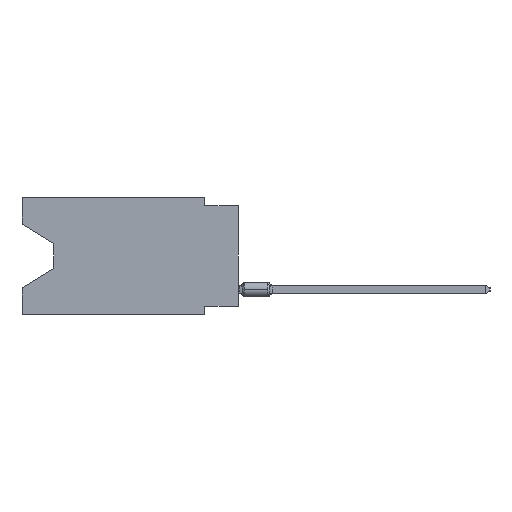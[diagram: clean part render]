
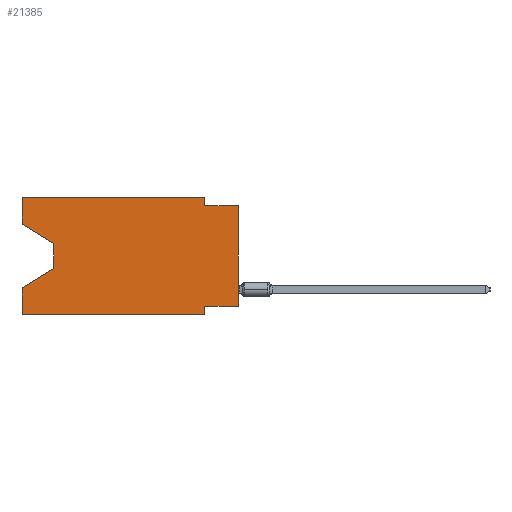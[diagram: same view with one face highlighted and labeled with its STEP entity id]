
A CAD part, left-side view. The second image highlights one B-rep face of the part: STEP entity #21385.
In plain terms, the highlighted planar face has unit normal (-1, 0, 0).
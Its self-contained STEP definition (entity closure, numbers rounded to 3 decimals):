
#199 = VECTOR ( 'NONE', #45842, 1000. ) ;
#416 = DIRECTION ( 'NONE',  ( 1., 0., 0. ) ) ;
#515 = ORIENTED_EDGE ( 'NONE', *, *, #51809, .F. ) ;
#555 = ORIENTED_EDGE ( 'NONE', *, *, #45054, .F. ) ;
#804 = CARTESIAN_POINT ( 'NONE',  ( 0., 16.383, 0. ) ) ;
#1162 = VERTEX_POINT ( 'NONE', #34680 ) ;
#1361 = DIRECTION ( 'NONE',  ( 0., 0., 1. ) ) ;
#1737 = EDGE_CURVE ( 'NONE', #40286, #1162, #40744, .T. ) ;
#2355 = VECTOR ( 'NONE', #50678, 1000. ) ;
#4151 = DIRECTION ( 'NONE',  ( 0., 0., -1. ) ) ;
#4203 = DIRECTION ( 'NONE',  ( 0., 0., 1. ) ) ;
#4494 = CARTESIAN_POINT ( 'NONE',  ( 0., 13.97, -5.385 ) ) ;
#4905 = CARTESIAN_POINT ( 'NONE',  ( 0., 2.54, -8.89 ) ) ;
#4946 = VECTOR ( 'NONE', #25974, 1000. ) ;
#4986 = CARTESIAN_POINT ( 'NONE',  ( 0., 2.54, -0.635 ) ) ;
#5326 = DIRECTION ( 'NONE',  ( 0., -1., 0. ) ) ;
#6406 = LINE ( 'NONE', #15173, #2355 ) ;
#9459 = VERTEX_POINT ( 'NONE', #20965 ) ;
#13341 = DIRECTION ( 'NONE',  ( 0., 1., 0. ) ) ;
#13420 = VERTEX_POINT ( 'NONE', #39479 ) ;
#13816 = LINE ( 'NONE', #26316, #24808 ) ;
#13938 = VECTOR ( 'NONE', #5326, 1000. ) ;
#14042 = EDGE_CURVE ( 'NONE', #21015, #50200, #6406, .T. ) ;
#14538 = CARTESIAN_POINT ( 'NONE',  ( 0., 13.97, -3.505 ) ) ;
#14725 = CARTESIAN_POINT ( 'NONE',  ( 0., 16.383, -8.89 ) ) ;
#15173 = CARTESIAN_POINT ( 'NONE',  ( 0., 13.97, -5.385 ) ) ;
#15688 = VERTEX_POINT ( 'NONE', #4986 ) ;
#15832 = VERTEX_POINT ( 'NONE', #14538 ) ;
#15868 = CARTESIAN_POINT ( 'NONE',  ( 0., 16.383, 0. ) ) ;
#16449 = CARTESIAN_POINT ( 'NONE',  ( 0., 0., 0. ) ) ;
#17050 = DIRECTION ( 'NONE',  ( 0., -1., 0. ) ) ;
#17174 = VECTOR ( 'NONE', #1361, 1000. ) ;
#17615 = ORIENTED_EDGE ( 'NONE', *, *, #14042, .T. ) ;
#18483 = VERTEX_POINT ( 'NONE', #27683 ) ;
#20035 = EDGE_LOOP ( 'NONE', ( #32592, #42545, #17615, #555, #37179, #515, #31273, #36219, #41719, #29268, #30513, #52200 ) ) ;
#20965 = CARTESIAN_POINT ( 'NONE',  ( 0., 2.54, 0. ) ) ;
#21015 = VERTEX_POINT ( 'NONE', #4494 ) ;
#21385 = ADVANCED_FACE ( 'NONE', ( #40959 ), #31877, .F. ) ;
#21562 = DIRECTION ( 'NONE',  ( 0., -1., 0. ) ) ;
#21571 = CARTESIAN_POINT ( 'NONE',  ( 0., 13.97, -3.505 ) ) ;
#22695 = DIRECTION ( 'NONE',  ( 0., -0.855, -0.519 ) ) ;
#22816 = CARTESIAN_POINT ( 'NONE',  ( 0., 0., -8.255 ) ) ;
#24808 = VECTOR ( 'NONE', #21562, 1000. ) ;
#25974 = DIRECTION ( 'NONE',  ( 0., 0., -1. ) ) ;
#26091 = LINE ( 'NONE', #804, #27036 ) ;
#26316 = CARTESIAN_POINT ( 'NONE',  ( 0., 0., -0.635 ) ) ;
#26979 = EDGE_CURVE ( 'NONE', #52168, #15832, #50711, .T. ) ;
#27036 = VECTOR ( 'NONE', #17050, 1000. ) ;
#27371 = CARTESIAN_POINT ( 'NONE',  ( 0., 16.383, -6.852 ) ) ;
#27683 = CARTESIAN_POINT ( 'NONE',  ( 0., 16.383, 0. ) ) ;
#29040 = VECTOR ( 'NONE', #13341, 1000. ) ;
#29268 = ORIENTED_EDGE ( 'NONE', *, *, #49001, .F. ) ;
#29567 = LINE ( 'NONE', #21571, #199 ) ;
#30376 = CARTESIAN_POINT ( 'NONE',  ( 0., 16.383, 0. ) ) ;
#30513 = ORIENTED_EDGE ( 'NONE', *, *, #48175, .F. ) ;
#31056 = DIRECTION ( 'NONE',  ( 0., 0., -1. ) ) ;
#31273 = ORIENTED_EDGE ( 'NONE', *, *, #35083, .F. ) ;
#31566 = VECTOR ( 'NONE', #31056, 1000. ) ;
#31840 = LINE ( 'NONE', #43879, #31566 ) ;
#31877 = PLANE ( 'NONE',  #42695 ) ;
#32592 = ORIENTED_EDGE ( 'NONE', *, *, #26979, .T. ) ;
#33045 = VECTOR ( 'NONE', #4203, 1000. ) ;
#34025 = EDGE_CURVE ( 'NONE', #52168, #18483, #50661, .T. ) ;
#34680 = CARTESIAN_POINT ( 'NONE',  ( 0., 0., -0.635 ) ) ;
#35083 = EDGE_CURVE ( 'NONE', #40286, #13420, #49348, .T. ) ;
#35620 = EDGE_CURVE ( 'NONE', #15688, #1162, #13816, .T. ) ;
#36219 = ORIENTED_EDGE ( 'NONE', *, *, #1737, .T. ) ;
#36380 = VERTEX_POINT ( 'NONE', #4905 ) ;
#36592 = VERTEX_POINT ( 'NONE', #14725 ) ;
#36738 = EDGE_CURVE ( 'NONE', #15832, #21015, #29567, .T. ) ;
#36834 = CARTESIAN_POINT ( 'NONE',  ( 0., 0., -8.255 ) ) ;
#37062 = CARTESIAN_POINT ( 'NONE',  ( 0., 16.383, 0. ) ) ;
#37179 = ORIENTED_EDGE ( 'NONE', *, *, #45653, .T. ) ;
#38190 = CARTESIAN_POINT ( 'NONE',  ( 0., 16.383, -2.038 ) ) ;
#39479 = CARTESIAN_POINT ( 'NONE',  ( 0., 2.54, -8.255 ) ) ;
#40286 = VERTEX_POINT ( 'NONE', #22816 ) ;
#40744 = LINE ( 'NONE', #16449, #33045 ) ;
#40959 = FACE_OUTER_BOUND ( 'NONE', #20035, .T. ) ;
#41719 = ORIENTED_EDGE ( 'NONE', *, *, #35620, .F. ) ;
#42545 = ORIENTED_EDGE ( 'NONE', *, *, #36738, .T. ) ;
#42695 = AXIS2_PLACEMENT_3D ( 'NONE', #15868, #416, #4151 ) ;
#43052 = CARTESIAN_POINT ( 'NONE',  ( 0., 2.54, 0. ) ) ;
#43694 = VECTOR ( 'NONE', #52751, 1000. ) ;
#43825 = CARTESIAN_POINT ( 'NONE',  ( 0., 16.383, -2.038 ) ) ;
#43879 = CARTESIAN_POINT ( 'NONE',  ( 0., 2.54, -8.89 ) ) ;
#45054 = EDGE_CURVE ( 'NONE', #36592, #50200, #49863, .T. ) ;
#45331 = LINE ( 'NONE', #46129, #13938 ) ;
#45653 = EDGE_CURVE ( 'NONE', #36592, #36380, #45331, .T. ) ;
#45842 = DIRECTION ( 'NONE',  ( 0., 0., -1. ) ) ;
#46129 = CARTESIAN_POINT ( 'NONE',  ( 0., 16.383, -8.89 ) ) ;
#48175 = EDGE_CURVE ( 'NONE', #18483, #9459, #26091, .T. ) ;
#48544 = VECTOR ( 'NONE', #22695, 1000. ) ;
#49001 = EDGE_CURVE ( 'NONE', #9459, #15688, #51306, .T. ) ;
#49348 = LINE ( 'NONE', #36834, #29040 ) ;
#49863 = LINE ( 'NONE', #37062, #43694 ) ;
#50200 = VERTEX_POINT ( 'NONE', #27371 ) ;
#50661 = LINE ( 'NONE', #30376, #17174 ) ;
#50678 = DIRECTION ( 'NONE',  ( 0., 0.855, -0.519 ) ) ;
#50711 = LINE ( 'NONE', #38190, #48544 ) ;
#51306 = LINE ( 'NONE', #43052, #4946 ) ;
#51809 = EDGE_CURVE ( 'NONE', #13420, #36380, #31840, .T. ) ;
#52168 = VERTEX_POINT ( 'NONE', #43825 ) ;
#52200 = ORIENTED_EDGE ( 'NONE', *, *, #34025, .F. ) ;
#52751 = DIRECTION ( 'NONE',  ( 0., 0., 1. ) ) ;
